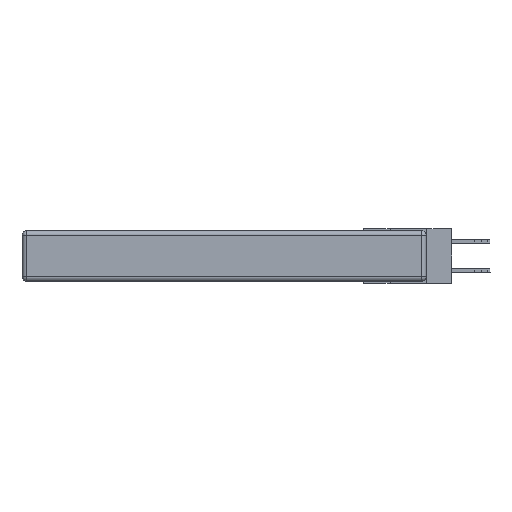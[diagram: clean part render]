
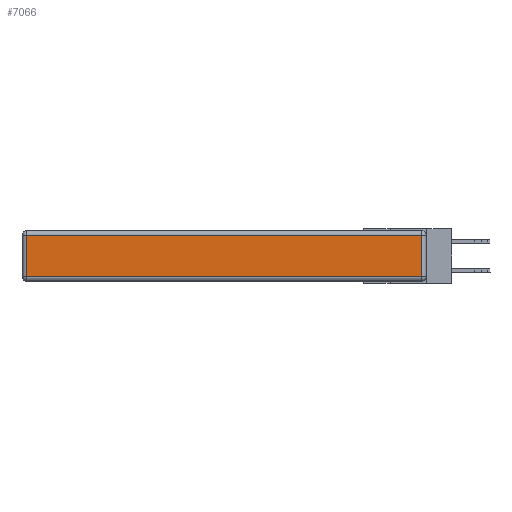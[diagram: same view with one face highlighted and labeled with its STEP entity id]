
A CAD part, left-side view. The second image highlights one B-rep face of the part: STEP entity #7066.
In plain terms, the highlighted planar face has unit normal (-1, 0, 0).
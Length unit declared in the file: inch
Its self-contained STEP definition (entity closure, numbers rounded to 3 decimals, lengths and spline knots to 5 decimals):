
#575 = VECTOR ( 'NONE', #9016, 39.37008 ) ;
#720 = VECTOR ( 'NONE', #11954, 39.37008 ) ;
#1224 = LINE ( 'NONE', #7948, #575 ) ;
#1614 = LINE ( 'NONE', #7530, #12665 ) ;
#1746 = EDGE_CURVE ( 'NONE', #11601, #6004, #1614, .T. ) ;
#2288 = FACE_OUTER_BOUND ( 'NONE', #9315, .T. ) ;
#2883 = DIRECTION ( 'NONE',  ( 0., -1., 0. ) ) ;
#4562 = PLANE ( 'NONE',  #9149 ) ;
#4658 = DIRECTION ( 'NONE',  ( 0., 0., 1. ) ) ;
#4765 = CARTESIAN_POINT ( 'NONE',  ( 0., 0.03, -0.313 ) ) ;
#5246 = ORIENTED_EDGE ( 'NONE', *, *, #8395, .T. ) ;
#5468 = VECTOR ( 'NONE', #2883, 39.37008 ) ;
#6004 = VERTEX_POINT ( 'NONE', #9352 ) ;
#6583 = DIRECTION ( 'NONE',  ( 0., 0., 1. ) ) ;
#7066 = ADVANCED_FACE ( 'NONE', ( #2288 ), #4562, .T. ) ;
#7530 = CARTESIAN_POINT ( 'NONE',  ( 0., 0.03, -0.343 ) ) ;
#7539 = LINE ( 'NONE', #10227, #5468 ) ;
#7704 = CARTESIAN_POINT ( 'NONE',  ( 0., 2.75, -0.03 ) ) ;
#7851 = CARTESIAN_POINT ( 'NONE',  ( 0., 0., -0.343 ) ) ;
#7948 = CARTESIAN_POINT ( 'NONE',  ( 0., 2.72, -0.343 ) ) ;
#8157 = ORIENTED_EDGE ( 'NONE', *, *, #8657, .T. ) ;
#8395 = EDGE_CURVE ( 'NONE', #6004, #9385, #11773, .T. ) ;
#8418 = CARTESIAN_POINT ( 'NONE',  ( 0., 2.72, -0.313 ) ) ;
#8657 = EDGE_CURVE ( 'NONE', #10979, #11601, #7539, .T. ) ;
#8700 = CARTESIAN_POINT ( 'NONE',  ( 0., 2.72, -0.03 ) ) ;
#8752 = ORIENTED_EDGE ( 'NONE', *, *, #1746, .T. ) ;
#8810 = EDGE_CURVE ( 'NONE', #9385, #10979, #1224, .T. ) ;
#9016 = DIRECTION ( 'NONE',  ( 0., 0., -1. ) ) ;
#9149 = AXIS2_PLACEMENT_3D ( 'NONE', #7851, #12983, #4658 ) ;
#9187 = ORIENTED_EDGE ( 'NONE', *, *, #8810, .T. ) ;
#9315 = EDGE_LOOP ( 'NONE', ( #8157, #8752, #5246, #9187 ) ) ;
#9352 = CARTESIAN_POINT ( 'NONE',  ( 0., 0.03, -0.03 ) ) ;
#9385 = VERTEX_POINT ( 'NONE', #8700 ) ;
#10227 = CARTESIAN_POINT ( 'NONE',  ( 0., 0., -0.313 ) ) ;
#10979 = VERTEX_POINT ( 'NONE', #8418 ) ;
#11601 = VERTEX_POINT ( 'NONE', #4765 ) ;
#11773 = LINE ( 'NONE', #7704, #720 ) ;
#11954 = DIRECTION ( 'NONE',  ( 0., 1., 0. ) ) ;
#12665 = VECTOR ( 'NONE', #6583, 39.37008 ) ;
#12983 = DIRECTION ( 'NONE',  ( -1., 0., 0. ) ) ;
